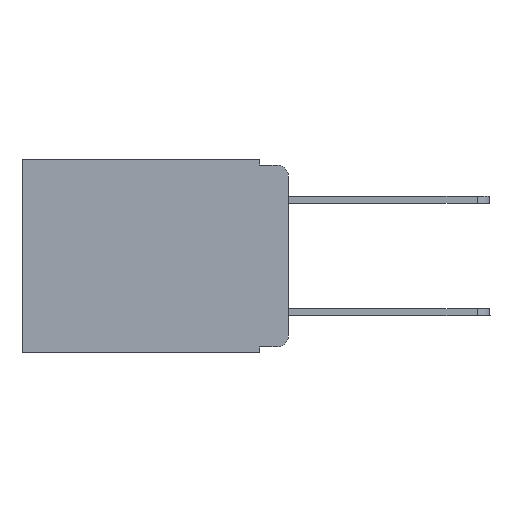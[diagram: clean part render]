
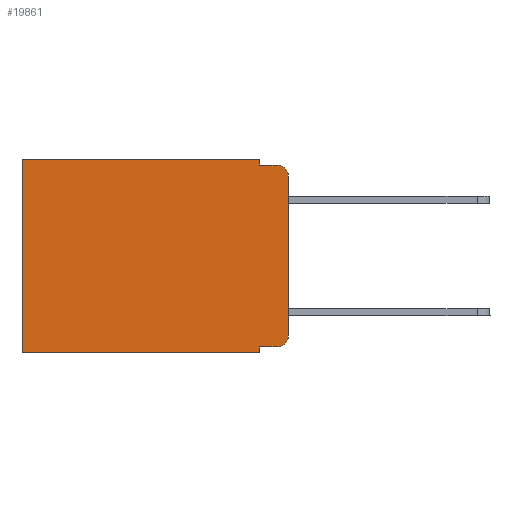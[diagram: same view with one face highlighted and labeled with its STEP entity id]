
A CAD part, left-side view. The second image highlights one B-rep face of the part: STEP entity #19861.
In plain terms, the highlighted planar face has unit normal (-1, 0, 0).
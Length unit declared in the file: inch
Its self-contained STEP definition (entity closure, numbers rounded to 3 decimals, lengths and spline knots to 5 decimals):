
#89 = VECTOR ( 'NONE', #2758, 39.37008 ) ;
#902 = CARTESIAN_POINT ( 'NONE',  ( 0.298, 0.051, 0. ) ) ;
#940 = VECTOR ( 'NONE', #14781, 39.37008 ) ;
#1001 = CARTESIAN_POINT ( 'NONE',  ( 0.298, 0.051, -0.333 ) ) ;
#1022 = CARTESIAN_POINT ( 'NONE',  ( 0.298, 0.051, -0.01 ) ) ;
#1198 = CIRCLE ( 'NONE', #17796, 0.02 ) ;
#1350 = DIRECTION ( 'NONE',  ( 0., 0., -1. ) ) ;
#1420 = DIRECTION ( 'NONE',  ( 1., 0., 0. ) ) ;
#1912 = CARTESIAN_POINT ( 'NONE',  ( 0.298, 0.02, -0.01 ) ) ;
#1984 = DIRECTION ( 'NONE',  ( 0., 0., -1. ) ) ;
#2121 = CARTESIAN_POINT ( 'NONE',  ( 0.298, 0.051, 0. ) ) ;
#2722 = DIRECTION ( 'NONE',  ( -1., 0., 0. ) ) ;
#2758 = DIRECTION ( 'NONE',  ( 0., 0., -1. ) ) ;
#2916 = LINE ( 'NONE', #1001, #14353 ) ;
#3087 = ORIENTED_EDGE ( 'NONE', *, *, #3381, .T. ) ;
#3381 = EDGE_CURVE ( 'NONE', #12431, #11439, #1198, .T. ) ;
#3971 = DIRECTION ( 'NONE',  ( 0., 0., -1. ) ) ;
#4235 = CARTESIAN_POINT ( 'NONE',  ( 0.298, 0.02, -0.03 ) ) ;
#4503 = EDGE_CURVE ( 'NONE', #17210, #5236, #12376, .T. ) ;
#4529 = CARTESIAN_POINT ( 'NONE',  ( 0.298, 0., -0.313 ) ) ;
#5101 = LINE ( 'NONE', #11511, #940 ) ;
#5236 = VERTEX_POINT ( 'NONE', #1912 ) ;
#5879 = ORIENTED_EDGE ( 'NONE', *, *, #10470, .T. ) ;
#6279 = VECTOR ( 'NONE', #15704, 39.37008 ) ;
#7143 = DIRECTION ( 'NONE',  ( 0., -1., 0. ) ) ;
#7484 = CARTESIAN_POINT ( 'NONE',  ( 0.298, 0.051, -0.01 ) ) ;
#7492 = ORIENTED_EDGE ( 'NONE', *, *, #13392, .F. ) ;
#7569 = VERTEX_POINT ( 'NONE', #7836 ) ;
#7696 = DIRECTION ( 'NONE',  ( 0., -1., 0. ) ) ;
#7767 = CARTESIAN_POINT ( 'NONE',  ( 0.298, 0.02, -0.333 ) ) ;
#7836 = CARTESIAN_POINT ( 'NONE',  ( 0.298, 0.051, -0.343 ) ) ;
#8128 = VERTEX_POINT ( 'NONE', #2121 ) ;
#8209 = VECTOR ( 'NONE', #7696, 39.37008 ) ;
#8305 = VERTEX_POINT ( 'NONE', #11698 ) ;
#9041 = CARTESIAN_POINT ( 'NONE',  ( 0.298, 0., 0. ) ) ;
#9253 = LINE ( 'NONE', #17365, #11718 ) ;
#10151 = VECTOR ( 'NONE', #15279, 39.37008 ) ;
#10399 = LINE ( 'NONE', #19939, #10151 ) ;
#10470 = EDGE_CURVE ( 'NONE', #12816, #12431, #2916, .T. ) ;
#10747 = ORIENTED_EDGE ( 'NONE', *, *, #12256, .F. ) ;
#10896 = EDGE_CURVE ( 'NONE', #8128, #8305, #5101, .T. ) ;
#10958 = EDGE_CURVE ( 'NONE', #11465, #5236, #15576, .T. ) ;
#11366 = EDGE_CURVE ( 'NONE', #7569, #11602, #10399, .T. ) ;
#11379 = EDGE_LOOP ( 'NONE', ( #12124, #18432, #14769, #7492, #14837, #14101, #17079, #10747, #5879, #3087 ) ) ;
#11439 = VERTEX_POINT ( 'NONE', #4529 ) ;
#11465 = VERTEX_POINT ( 'NONE', #20089 ) ;
#11511 = CARTESIAN_POINT ( 'NONE',  ( 0.298, 0., 0. ) ) ;
#11602 = VERTEX_POINT ( 'NONE', #15570 ) ;
#11698 = CARTESIAN_POINT ( 'NONE',  ( 0.298, 0.473, 0. ) ) ;
#11718 = VECTOR ( 'NONE', #14090, 39.37008 ) ;
#11930 = AXIS2_PLACEMENT_3D ( 'NONE', #4235, #15144, #1984 ) ;
#12124 = ORIENTED_EDGE ( 'NONE', *, *, #16693, .F. ) ;
#12162 = DIRECTION ( 'NONE',  ( 0., 0., -1. ) ) ;
#12256 = EDGE_CURVE ( 'NONE', #12816, #7569, #20180, .T. ) ;
#12376 = LINE ( 'NONE', #7484, #8209 ) ;
#12431 = VERTEX_POINT ( 'NONE', #7767 ) ;
#12611 = FACE_OUTER_BOUND ( 'NONE', #11379, .T. ) ;
#12816 = VERTEX_POINT ( 'NONE', #18206 ) ;
#13392 = EDGE_CURVE ( 'NONE', #8128, #17210, #19943, .T. ) ;
#14090 = DIRECTION ( 'NONE',  ( 0., 0., -1. ) ) ;
#14099 = CARTESIAN_POINT ( 'NONE',  ( 0.298, 0.02, -0.313 ) ) ;
#14101 = ORIENTED_EDGE ( 'NONE', *, *, #17397, .T. ) ;
#14353 = VECTOR ( 'NONE', #7143, 39.37008 ) ;
#14769 = ORIENTED_EDGE ( 'NONE', *, *, #4503, .F. ) ;
#14781 = DIRECTION ( 'NONE',  ( 0., 1., 0. ) ) ;
#14837 = ORIENTED_EDGE ( 'NONE', *, *, #10896, .T. ) ;
#14999 = CARTESIAN_POINT ( 'NONE',  ( 0.298, 0.051, 0. ) ) ;
#15144 = DIRECTION ( 'NONE',  ( -1., 0., 0. ) ) ;
#15279 = DIRECTION ( 'NONE',  ( 0., 1., 0. ) ) ;
#15320 = PLANE ( 'NONE',  #19899 ) ;
#15570 = CARTESIAN_POINT ( 'NONE',  ( 0.298, 0.473, -0.343 ) ) ;
#15576 = CIRCLE ( 'NONE', #11930, 0.02 ) ;
#15704 = DIRECTION ( 'NONE',  ( 0., 0., -1. ) ) ;
#16693 = EDGE_CURVE ( 'NONE', #11465, #11439, #17861, .T. ) ;
#17079 = ORIENTED_EDGE ( 'NONE', *, *, #11366, .F. ) ;
#17210 = VERTEX_POINT ( 'NONE', #1022 ) ;
#17365 = CARTESIAN_POINT ( 'NONE',  ( 0.298, 0.473, 0. ) ) ;
#17397 = EDGE_CURVE ( 'NONE', #8305, #11602, #9253, .T. ) ;
#17796 = AXIS2_PLACEMENT_3D ( 'NONE', #14099, #2722, #12162 ) ;
#17861 = LINE ( 'NONE', #9041, #89 ) ;
#18206 = CARTESIAN_POINT ( 'NONE',  ( 0.298, 0.051, -0.333 ) ) ;
#18432 = ORIENTED_EDGE ( 'NONE', *, *, #10958, .T. ) ;
#18534 = CARTESIAN_POINT ( 'NONE',  ( 0.298, 0., 0. ) ) ;
#19208 = VECTOR ( 'NONE', #3971, 39.37008 ) ;
#19861 = ADVANCED_FACE ( 'NONE', ( #12611 ), #15320, .F. ) ;
#19899 = AXIS2_PLACEMENT_3D ( 'NONE', #18534, #1420, #1350 ) ;
#19939 = CARTESIAN_POINT ( 'NONE',  ( 0.298, 0., -0.343 ) ) ;
#19943 = LINE ( 'NONE', #902, #6279 ) ;
#20089 = CARTESIAN_POINT ( 'NONE',  ( 0.298, 0., -0.03 ) ) ;
#20180 = LINE ( 'NONE', #14999, #19208 ) ;
